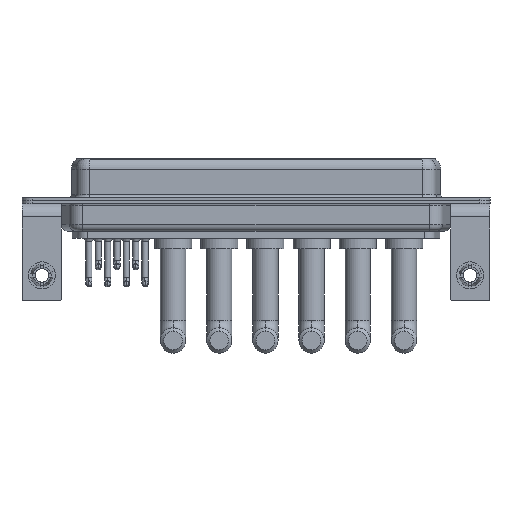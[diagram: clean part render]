
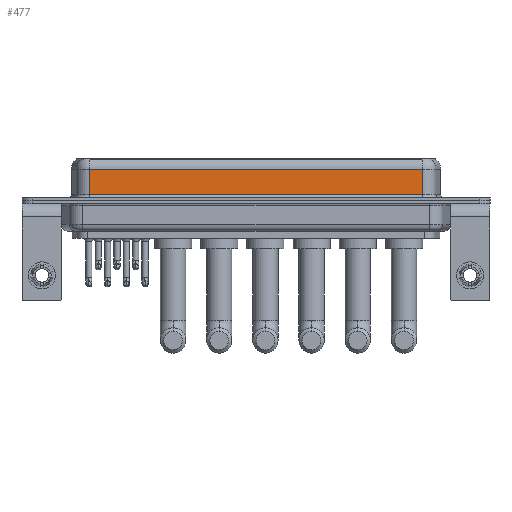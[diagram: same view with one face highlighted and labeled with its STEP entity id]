
A CAD part, front view. The second image highlights one B-rep face of the part: STEP entity #477.
In plain terms, the highlighted planar face has unit normal (0, -1, 0).
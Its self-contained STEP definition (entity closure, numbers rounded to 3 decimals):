
#468 = DIRECTION ( 'NONE',  ( 0., 0., 1. ) ) ;
#477 = ADVANCED_FACE ( 'NONE', ( #1425 ), #13118, .F. ) ;
#547 = ORIENTED_EDGE ( 'NONE', *, *, #10506, .T. ) ;
#904 = VERTEX_POINT ( 'NONE', #17937 ) ;
#962 = LINE ( 'NONE', #7407, #17685 ) ;
#1072 = CARTESIAN_POINT ( 'NONE',  ( 7.038, -3.95, 4.65 ) ) ;
#1235 = DIRECTION ( 'NONE',  ( -1., 0., 0. ) ) ;
#1301 = CARTESIAN_POINT ( 'NONE',  ( 7.038, -3.95, 0.9 ) ) ;
#1425 = FACE_OUTER_BOUND ( 'NONE', #12859, .T. ) ;
#1459 = CARTESIAN_POINT ( 'NONE',  ( 56.462, -3.95, 0.9 ) ) ;
#2976 = DIRECTION ( 'NONE',  ( 0., 0., -1. ) ) ;
#5432 = VERTEX_POINT ( 'NONE', #1301 ) ;
#6348 = ORIENTED_EDGE ( 'NONE', *, *, #14891, .T. ) ;
#6766 = CARTESIAN_POINT ( 'NONE',  ( 7.038, -3.95, 6.4 ) ) ;
#7059 = VERTEX_POINT ( 'NONE', #1072 ) ;
#7407 = CARTESIAN_POINT ( 'NONE',  ( 56.462, -3.95, 6.4 ) ) ;
#7565 = LINE ( 'NONE', #12402, #11433 ) ;
#7918 = VECTOR ( 'NONE', #9577, 1000. ) ;
#8912 = CARTESIAN_POINT ( 'NONE',  ( 56.462, -3.95, 4.65 ) ) ;
#9577 = DIRECTION ( 'NONE',  ( 1., 0., 0. ) ) ;
#10060 = VECTOR ( 'NONE', #18029, 1000. ) ;
#10506 = EDGE_CURVE ( 'NONE', #5432, #904, #15905, .T. ) ;
#11286 = EDGE_CURVE ( 'NONE', #16963, #904, #962, .T. ) ;
#11433 = VECTOR ( 'NONE', #1235, 1000. ) ;
#12402 = CARTESIAN_POINT ( 'NONE',  ( 56.462, -3.95, 4.65 ) ) ;
#12859 = EDGE_LOOP ( 'NONE', ( #19025, #6348, #14119, #547 ) ) ;
#13118 = PLANE ( 'NONE',  #19832 ) ;
#14119 = ORIENTED_EDGE ( 'NONE', *, *, #20205, .T. ) ;
#14805 = DIRECTION ( 'NONE',  ( 0., 1., 0. ) ) ;
#14891 = EDGE_CURVE ( 'NONE', #16963, #7059, #7565, .T. ) ;
#14969 = LINE ( 'NONE', #6766, #10060 ) ;
#15007 = CARTESIAN_POINT ( 'NONE',  ( 56.462, -3.95, 6.4 ) ) ;
#15905 = LINE ( 'NONE', #1459, #7918 ) ;
#16963 = VERTEX_POINT ( 'NONE', #8912 ) ;
#17685 = VECTOR ( 'NONE', #2976, 1000. ) ;
#17937 = CARTESIAN_POINT ( 'NONE',  ( 56.462, -3.95, 0.9 ) ) ;
#18029 = DIRECTION ( 'NONE',  ( 0., 0., -1. ) ) ;
#19025 = ORIENTED_EDGE ( 'NONE', *, *, #11286, .F. ) ;
#19832 = AXIS2_PLACEMENT_3D ( 'NONE', #15007, #14805, #468 ) ;
#20205 = EDGE_CURVE ( 'NONE', #7059, #5432, #14969, .T. ) ;
